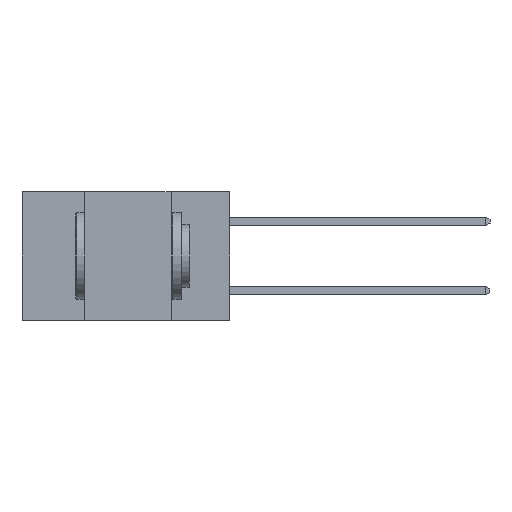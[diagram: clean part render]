
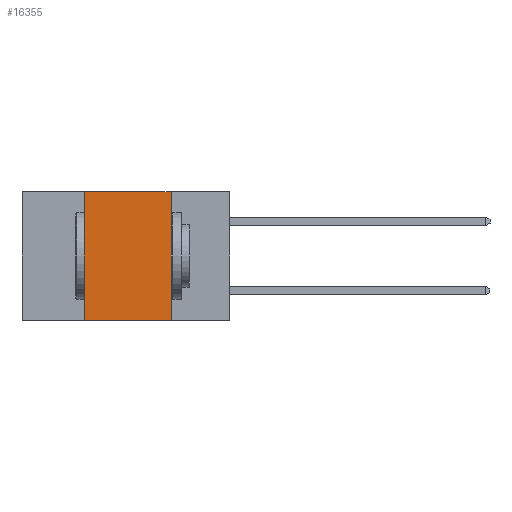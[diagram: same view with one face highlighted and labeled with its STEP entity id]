
A CAD part, left-side view. The second image highlights one B-rep face of the part: STEP entity #16355.
In plain terms, the highlighted planar face has unit normal (-1, 0, 0).
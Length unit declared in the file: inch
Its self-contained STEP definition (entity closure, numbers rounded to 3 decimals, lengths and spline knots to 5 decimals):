
#395 = VECTOR ( 'NONE', #26373, 39.37008 ) ;
#2263 = DIRECTION ( 'NONE',  ( 1., 0., 0. ) ) ;
#3454 = EDGE_CURVE ( 'NONE', #7892, #25791, #20178, .T. ) ;
#4367 = LINE ( 'NONE', #17350, #22577 ) ;
#4448 = ORIENTED_EDGE ( 'NONE', *, *, #20693, .F. ) ;
#5412 = AXIS2_PLACEMENT_3D ( 'NONE', #31970, #2263, #19633 ) ;
#5610 = VECTOR ( 'NONE', #11796, 39.37008 ) ;
#5647 = EDGE_LOOP ( 'NONE', ( #4448, #5987, #6759, #26169 ) ) ;
#5698 = VECTOR ( 'NONE', #15098, 39.37008 ) ;
#5710 = EDGE_CURVE ( 'NONE', #7892, #25966, #32078, .T. ) ;
#5987 = ORIENTED_EDGE ( 'NONE', *, *, #7095, .F. ) ;
#6759 = ORIENTED_EDGE ( 'NONE', *, *, #5710, .F. ) ;
#7095 = EDGE_CURVE ( 'NONE', #25966, #9977, #18826, .T. ) ;
#7607 = CARTESIAN_POINT ( 'NONE',  ( 0., 0.6, -0.37 ) ) ;
#7892 = VERTEX_POINT ( 'NONE', #12299 ) ;
#9260 = CARTESIAN_POINT ( 'NONE',  ( 0., 0.6, 0. ) ) ;
#9977 = VERTEX_POINT ( 'NONE', #26233 ) ;
#11796 = DIRECTION ( 'NONE',  ( 0., -1., 0. ) ) ;
#12299 = CARTESIAN_POINT ( 'NONE',  ( 0., 0.42, -0.37 ) ) ;
#14624 = PLANE ( 'NONE',  #5412 ) ;
#15098 = DIRECTION ( 'NONE',  ( 0., 0., 1. ) ) ;
#16355 = ADVANCED_FACE ( 'NONE', ( #27949 ), #14624, .F. ) ;
#17350 = CARTESIAN_POINT ( 'NONE',  ( 0., 0.17, 0. ) ) ;
#17446 = CARTESIAN_POINT ( 'NONE',  ( 0., 0.42, 0. ) ) ;
#18826 = LINE ( 'NONE', #9260, #5610 ) ;
#19633 = DIRECTION ( 'NONE',  ( 0., 0., -1. ) ) ;
#19853 = DIRECTION ( 'NONE',  ( 0., 0., -1. ) ) ;
#20178 = LINE ( 'NONE', #7607, #395 ) ;
#20693 = EDGE_CURVE ( 'NONE', #9977, #25791, #4367, .T. ) ;
#22577 = VECTOR ( 'NONE', #19853, 39.37008 ) ;
#25791 = VERTEX_POINT ( 'NONE', #31522 ) ;
#25966 = VERTEX_POINT ( 'NONE', #27276 ) ;
#26169 = ORIENTED_EDGE ( 'NONE', *, *, #3454, .T. ) ;
#26233 = CARTESIAN_POINT ( 'NONE',  ( 0., 0.17, 0. ) ) ;
#26373 = DIRECTION ( 'NONE',  ( 0., -1., 0. ) ) ;
#27276 = CARTESIAN_POINT ( 'NONE',  ( 0., 0.42, 0. ) ) ;
#27949 = FACE_OUTER_BOUND ( 'NONE', #5647, .T. ) ;
#31522 = CARTESIAN_POINT ( 'NONE',  ( 0., 0.17, -0.37 ) ) ;
#31970 = CARTESIAN_POINT ( 'NONE',  ( 0., 0.6, 0. ) ) ;
#32078 = LINE ( 'NONE', #17446, #5698 ) ;
